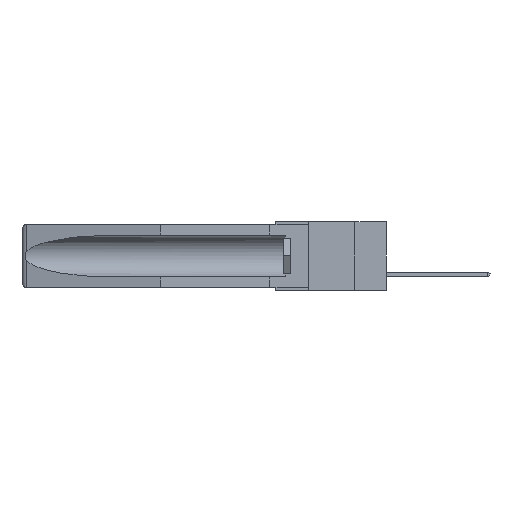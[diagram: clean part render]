
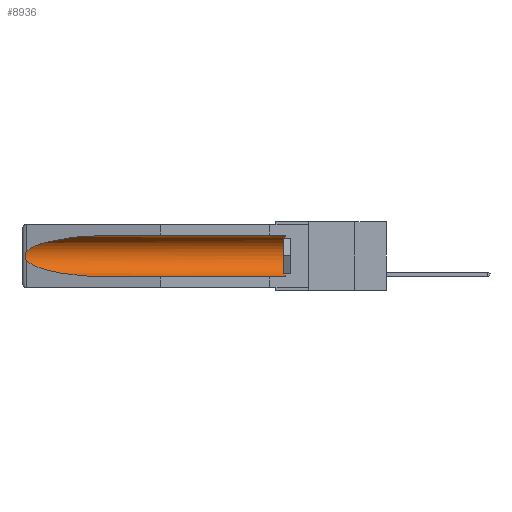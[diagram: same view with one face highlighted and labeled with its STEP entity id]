
A CAD part, left-side view. The second image highlights one B-rep face of the part: STEP entity #8936.
In plain terms, the highlighted cylindrical face has radius 2.857 mm (diameter 5.715 mm), a partial arc.
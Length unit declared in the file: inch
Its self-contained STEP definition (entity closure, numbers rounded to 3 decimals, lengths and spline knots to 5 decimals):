
#851 = CARTESIAN_POINT ( 'NONE',  ( 0.21114, 1.30732, -0.059 ) ) ;
#1075 = CIRCLE ( 'NONE', #18831, 0.1125 ) ;
#1312 = CARTESIAN_POINT ( 'NONE',  ( 0.26597, 1.52961, -0.15275 ) ) ;
#1426 = ORIENTED_EDGE ( 'NONE', *, *, #10948, .T. ) ;
#1935 = EDGE_CURVE ( 'NONE', #14154, #15611, #6321, .T. ) ;
#2859 = VERTEX_POINT ( 'NONE', #16480 ) ;
#3303 = CARTESIAN_POINT ( 'NONE',  ( 0.155, 1.07973, -0.284 ) ) ;
#3578 = AXIS2_PLACEMENT_3D ( 'NONE', #3890, #12605, #15682 ) ;
#3890 = CARTESIAN_POINT ( 'NONE',  ( 0.155, -0.30754, -0.1715 ) ) ;
#4083 = EDGE_CURVE ( 'NONE', #5126, #2859, #16354, .T. ) ;
#4175 = CARTESIAN_POINT ( 'NONE',  ( 0.2675, 1.53308, -0.17534 ) ) ;
#5059 = CARTESIAN_POINT ( 'NONE',  ( 0.25451, 1.48313, -0.09465 ) ) ;
#5126 = VERTEX_POINT ( 'NONE', #5336 ) ;
#5336 = CARTESIAN_POINT ( 'NONE',  ( 0.26537, 1.52718, -0.19328 ) ) ;
#5591 = CARTESIAN_POINT ( 'NONE',  ( 0.26537, 1.52718, -0.19328 ) ) ;
#5609 = LINE ( 'NONE', #7316, #13443 ) ;
#6321 =( BOUNDED_CURVE ( )  B_SPLINE_CURVE ( 3, ( #9507, #851, #5059, #6735 ),
 .UNSPECIFIED., .F., .F. ) 
 B_SPLINE_CURVE_WITH_KNOTS ( ( 4, 4 ),
 ( 4.71239, 6.08839 ),
 .UNSPECIFIED. ) 
 CURVE ( )  GEOMETRIC_REPRESENTATION_ITEM ( )  RATIONAL_B_SPLINE_CURVE ( ( 1., 0.848, 0.848, 1. ) ) 
 REPRESENTATION_ITEM ( '' )  );
#6735 = CARTESIAN_POINT ( 'NONE',  ( 0.26537, 1.52718, -0.14972 ) ) ;
#6834 = DIRECTION ( 'NONE',  ( 0., -1., 0. ) ) ;
#7035 = CARTESIAN_POINT ( 'NONE',  ( 0.155, 0.126, -0.1715 ) ) ;
#7308 = ORIENTED_EDGE ( 'NONE', *, *, #15952, .T. ) ;
#7316 = CARTESIAN_POINT ( 'NONE',  ( 0.155, -0.30754, -0.059 ) ) ;
#7968 = CARTESIAN_POINT ( 'NONE',  ( 0.155, 0.126, -0.059 ) ) ;
#8445 = DIRECTION ( 'NONE',  ( 0., 1., 0. ) ) ;
#8589 = ORIENTED_EDGE ( 'NONE', *, *, #13231, .F. ) ;
#8727 = CARTESIAN_POINT ( 'NONE',  ( 0.2675, 1.53308, -0.16763 ) ) ;
#8936 = ADVANCED_FACE ( 'NONE', ( #12613 ), #9831, .F. ) ;
#9060 = CARTESIAN_POINT ( 'NONE',  ( 0.21114, 1.30732, -0.284 ) ) ;
#9413 = CARTESIAN_POINT ( 'NONE',  ( 0.155, 0.126, -0.284 ) ) ;
#9507 = CARTESIAN_POINT ( 'NONE',  ( 0.155, 1.07973, -0.059 ) ) ;
#9831 = CYLINDRICAL_SURFACE ( 'NONE', #3578, 0.1125 ) ;
#9935 = CARTESIAN_POINT ( 'NONE',  ( 0.155, -0.30754, -0.284 ) ) ;
#10023 = CARTESIAN_POINT ( 'NONE',  ( 0.26655, 1.53094, -0.18657 ) ) ;
#10412 = VERTEX_POINT ( 'NONE', #7968 ) ;
#10572 = CARTESIAN_POINT ( 'NONE',  ( 0.155, 1.07973, -0.059 ) ) ;
#10948 = EDGE_CURVE ( 'NONE', #10412, #14154, #5609, .T. ) ;
#11040 = B_SPLINE_CURVE_WITH_KNOTS ( 'NONE', 3,
 ( #19108, #1312, #11695, #17567, #8727, #4175, #13069, #10023, #15947, #5591 ),
 .UNSPECIFIED., .F., .F.,
 ( 4, 2, 2, 2, 4 ),
 ( 0., 0.00029, 0.00058, 0.00087, 0.00117 ),
 .UNSPECIFIED. ) ;
#11610 = VERTEX_POINT ( 'NONE', #9413 ) ;
#11695 = CARTESIAN_POINT ( 'NONE',  ( 0.26654, 1.53092, -0.15636 ) ) ;
#12012 = CARTESIAN_POINT ( 'NONE',  ( 0.25451, 1.48313, -0.24835 ) ) ;
#12605 = DIRECTION ( 'NONE',  ( 0., 1., 0. ) ) ;
#12613 = FACE_OUTER_BOUND ( 'NONE', #15308, .T. ) ;
#12715 = LINE ( 'NONE', #9935, #15474 ) ;
#12978 = EDGE_CURVE ( 'NONE', #15611, #5126, #11040, .T. ) ;
#13069 = CARTESIAN_POINT ( 'NONE',  ( 0.2673, 1.53269, -0.17917 ) ) ;
#13231 = EDGE_CURVE ( 'NONE', #11610, #2859, #12715, .T. ) ;
#13443 = VECTOR ( 'NONE', #17613, 39.37008 ) ;
#13777 = ORIENTED_EDGE ( 'NONE', *, *, #12978, .T. ) ;
#13982 = ORIENTED_EDGE ( 'NONE', *, *, #4083, .T. ) ;
#14154 = VERTEX_POINT ( 'NONE', #10572 ) ;
#15308 = EDGE_LOOP ( 'NONE', ( #15499, #13777, #13982, #8589, #7308, #1426 ) ) ;
#15474 = VECTOR ( 'NONE', #8445, 39.37008 ) ;
#15499 = ORIENTED_EDGE ( 'NONE', *, *, #1935, .T. ) ;
#15611 = VERTEX_POINT ( 'NONE', #17861 ) ;
#15682 = DIRECTION ( 'NONE',  ( 0., 0., 1. ) ) ;
#15947 = CARTESIAN_POINT ( 'NONE',  ( 0.26597, 1.5296, -0.19026 ) ) ;
#15952 = EDGE_CURVE ( 'NONE', #11610, #10412, #1075, .T. ) ;
#16354 =( BOUNDED_CURVE ( )  B_SPLINE_CURVE ( 3, ( #16377, #12012, #9060, #3303 ),
 .UNSPECIFIED., .F., .F. ) 
 B_SPLINE_CURVE_WITH_KNOTS ( ( 4, 4 ),
 ( 0.1948, 1.5708 ),
 .UNSPECIFIED. ) 
 CURVE ( )  GEOMETRIC_REPRESENTATION_ITEM ( )  RATIONAL_B_SPLINE_CURVE ( ( 1., 0.848, 0.848, 1. ) ) 
 REPRESENTATION_ITEM ( '' )  );
#16377 = CARTESIAN_POINT ( 'NONE',  ( 0.26537, 1.52718, -0.19328 ) ) ;
#16480 = CARTESIAN_POINT ( 'NONE',  ( 0.155, 1.07973, -0.284 ) ) ;
#17198 = DIRECTION ( 'NONE',  ( 0., 0., 1. ) ) ;
#17567 = CARTESIAN_POINT ( 'NONE',  ( 0.2673, 1.5327, -0.16383 ) ) ;
#17613 = DIRECTION ( 'NONE',  ( 0., 1., 0. ) ) ;
#17861 = CARTESIAN_POINT ( 'NONE',  ( 0.26537, 1.52718, -0.14972 ) ) ;
#18831 = AXIS2_PLACEMENT_3D ( 'NONE', #7035, #6834, #17198 ) ;
#19108 = CARTESIAN_POINT ( 'NONE',  ( 0.26537, 1.52718, -0.14972 ) ) ;
